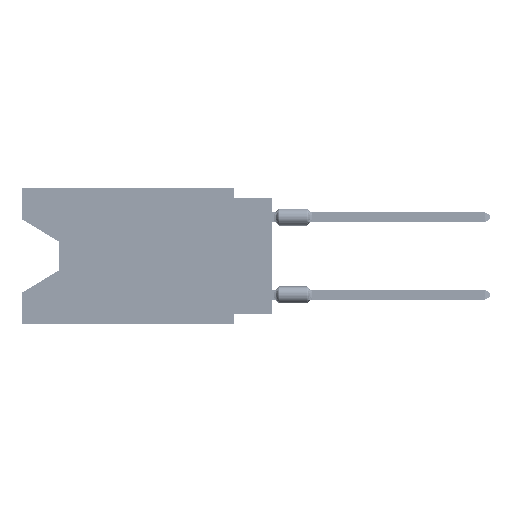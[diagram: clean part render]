
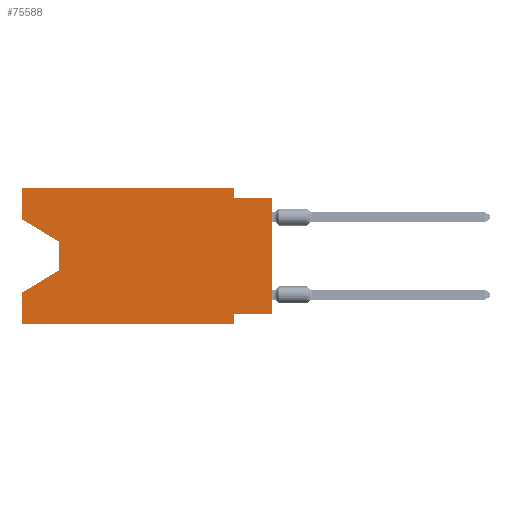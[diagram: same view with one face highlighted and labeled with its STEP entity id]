
A CAD part, left-side view. The second image highlights one B-rep face of the part: STEP entity #75588.
In plain terms, the highlighted planar face has unit normal (-1, 0, 0).
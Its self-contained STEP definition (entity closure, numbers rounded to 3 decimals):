
#758 = DIRECTION ( 'NONE',  ( 0., 0., -1. ) ) ;
#1873 = CARTESIAN_POINT ( 'NONE',  ( 0., 16.383, -8.89 ) ) ;
#2846 = ORIENTED_EDGE ( 'NONE', *, *, #29020, .F. ) ;
#3597 = LINE ( 'NONE', #11110, #65106 ) ;
#3714 = CARTESIAN_POINT ( 'NONE',  ( 0., 13.97, -5.385 ) ) ;
#6676 = VERTEX_POINT ( 'NONE', #95369 ) ;
#7500 = CARTESIAN_POINT ( 'NONE',  ( 0., 13.97, -3.505 ) ) ;
#9991 = CARTESIAN_POINT ( 'NONE',  ( 0., 16.383, 0. ) ) ;
#10137 = LINE ( 'NONE', #45891, #101192 ) ;
#11110 = CARTESIAN_POINT ( 'NONE',  ( 0., 16.383, -2.038 ) ) ;
#13546 = VERTEX_POINT ( 'NONE', #1873 ) ;
#13571 = CARTESIAN_POINT ( 'NONE',  ( 0., 16.383, -6.852 ) ) ;
#15167 = ORIENTED_EDGE ( 'NONE', *, *, #69775, .F. ) ;
#16075 = CARTESIAN_POINT ( 'NONE',  ( 0., 16.383, 0. ) ) ;
#16445 = EDGE_CURVE ( 'NONE', #98619, #56858, #60688, .T. ) ;
#16849 = DIRECTION ( 'NONE',  ( 0., 0., -1. ) ) ;
#18128 = ORIENTED_EDGE ( 'NONE', *, *, #16445, .T. ) ;
#18878 = DIRECTION ( 'NONE',  ( 0., 0., -1. ) ) ;
#21071 = DIRECTION ( 'NONE',  ( 0., 0., 1. ) ) ;
#21631 = VECTOR ( 'NONE', #18878, 1000. ) ;
#24177 = LINE ( 'NONE', #111835, #88287 ) ;
#24714 = DIRECTION ( 'NONE',  ( 0., -1., 0. ) ) ;
#25618 = VECTOR ( 'NONE', #24714, 1000. ) ;
#26440 = DIRECTION ( 'NONE',  ( 0., 0., 1. ) ) ;
#26732 = CARTESIAN_POINT ( 'NONE',  ( 0., 13.97, -5.385 ) ) ;
#27245 = CARTESIAN_POINT ( 'NONE',  ( 0., 16.383, 0. ) ) ;
#27459 = LINE ( 'NONE', #36098, #98020 ) ;
#29020 = EDGE_CURVE ( 'NONE', #13546, #40004, #30423, .T. ) ;
#30423 = LINE ( 'NONE', #41899, #40083 ) ;
#30498 = VERTEX_POINT ( 'NONE', #62076 ) ;
#30545 = EDGE_CURVE ( 'NONE', #84445, #42685, #10137, .T. ) ;
#30746 = VECTOR ( 'NONE', #26440, 1000. ) ;
#30876 = LINE ( 'NONE', #56811, #97747 ) ;
#34807 = ORIENTED_EDGE ( 'NONE', *, *, #102158, .T. ) ;
#36098 = CARTESIAN_POINT ( 'NONE',  ( 0., 0., -0.635 ) ) ;
#37066 = PLANE ( 'NONE',  #46306 ) ;
#37326 = EDGE_CURVE ( 'NONE', #68299, #98619, #3597, .T. ) ;
#37914 = VECTOR ( 'NONE', #95426, 1000. ) ;
#40004 = VERTEX_POINT ( 'NONE', #13571 ) ;
#40083 = VECTOR ( 'NONE', #101930, 1000. ) ;
#40901 = CARTESIAN_POINT ( 'NONE',  ( 0., 0., -0.635 ) ) ;
#41551 = EDGE_CURVE ( 'NONE', #68299, #113797, #50683, .T. ) ;
#41899 = CARTESIAN_POINT ( 'NONE',  ( 0., 16.383, 0. ) ) ;
#42685 = VERTEX_POINT ( 'NONE', #40901 ) ;
#44831 = VECTOR ( 'NONE', #16849, 1000. ) ;
#45407 = CARTESIAN_POINT ( 'NONE',  ( 0., 2.54, 0. ) ) ;
#45891 = CARTESIAN_POINT ( 'NONE',  ( 0., 0., 0. ) ) ;
#46096 = EDGE_CURVE ( 'NONE', #110345, #42685, #27459, .T. ) ;
#46296 = DIRECTION ( 'NONE',  ( 0., -0.855, -0.519 ) ) ;
#46306 = AXIS2_PLACEMENT_3D ( 'NONE', #9991, #90161, #758 ) ;
#50683 = LINE ( 'NONE', #16075, #30746 ) ;
#53201 = LINE ( 'NONE', #88431, #101116 ) ;
#56811 = CARTESIAN_POINT ( 'NONE',  ( 0., 2.54, -8.89 ) ) ;
#56858 = VERTEX_POINT ( 'NONE', #3714 ) ;
#56891 = ORIENTED_EDGE ( 'NONE', *, *, #66523, .T. ) ;
#60211 = LINE ( 'NONE', #26732, #37914 ) ;
#60212 = CARTESIAN_POINT ( 'NONE',  ( 0., 2.54, -0.635 ) ) ;
#60461 = VERTEX_POINT ( 'NONE', #82887 ) ;
#60688 = LINE ( 'NONE', #95908, #44831 ) ;
#62076 = CARTESIAN_POINT ( 'NONE',  ( 0., 2.54, -8.89 ) ) ;
#62352 = ORIENTED_EDGE ( 'NONE', *, *, #46096, .F. ) ;
#63884 = EDGE_CURVE ( 'NONE', #6676, #30498, #30876, .T. ) ;
#65106 = VECTOR ( 'NONE', #46296, 1000. ) ;
#66523 = EDGE_CURVE ( 'NONE', #56858, #40004, #60211, .T. ) ;
#68299 = VERTEX_POINT ( 'NONE', #82518 ) ;
#69775 = EDGE_CURVE ( 'NONE', #60461, #110345, #107678, .T. ) ;
#75588 = ADVANCED_FACE ( 'NONE', ( #81509 ), #37066, .F. ) ;
#77019 = EDGE_LOOP ( 'NONE', ( #101471, #18128, #56891, #2846, #34807, #110841, #83288, #77385, #62352, #15167, #92403, #94935 ) ) ;
#77385 = ORIENTED_EDGE ( 'NONE', *, *, #30545, .T. ) ;
#77781 = CARTESIAN_POINT ( 'NONE',  ( 0., 16.383, 0. ) ) ;
#80867 = EDGE_CURVE ( 'NONE', #84445, #6676, #53201, .T. ) ;
#81509 = FACE_OUTER_BOUND ( 'NONE', #77019, .T. ) ;
#82518 = CARTESIAN_POINT ( 'NONE',  ( 0., 16.383, -2.038 ) ) ;
#82887 = CARTESIAN_POINT ( 'NONE',  ( 0., 2.54, 0. ) ) ;
#83288 = ORIENTED_EDGE ( 'NONE', *, *, #80867, .F. ) ;
#84445 = VERTEX_POINT ( 'NONE', #107425 ) ;
#86438 = LINE ( 'NONE', #77781, #25618 ) ;
#87631 = DIRECTION ( 'NONE',  ( 0., -1., 0. ) ) ;
#88287 = VECTOR ( 'NONE', #87631, 1000. ) ;
#88431 = CARTESIAN_POINT ( 'NONE',  ( 0., 0., -8.255 ) ) ;
#90161 = DIRECTION ( 'NONE',  ( 1., 0., 0. ) ) ;
#90915 = EDGE_CURVE ( 'NONE', #113797, #60461, #86438, .T. ) ;
#91469 = DIRECTION ( 'NONE',  ( 0., 0., -1. ) ) ;
#92403 = ORIENTED_EDGE ( 'NONE', *, *, #90915, .F. ) ;
#94935 = ORIENTED_EDGE ( 'NONE', *, *, #41551, .F. ) ;
#95369 = CARTESIAN_POINT ( 'NONE',  ( 0., 2.54, -8.255 ) ) ;
#95426 = DIRECTION ( 'NONE',  ( 0., 0.855, -0.519 ) ) ;
#95908 = CARTESIAN_POINT ( 'NONE',  ( 0., 13.97, -3.505 ) ) ;
#97747 = VECTOR ( 'NONE', #91469, 1000. ) ;
#98020 = VECTOR ( 'NONE', #105358, 1000. ) ;
#98619 = VERTEX_POINT ( 'NONE', #7500 ) ;
#98761 = DIRECTION ( 'NONE',  ( 0., 1., 0. ) ) ;
#101116 = VECTOR ( 'NONE', #98761, 1000. ) ;
#101192 = VECTOR ( 'NONE', #21071, 1000. ) ;
#101471 = ORIENTED_EDGE ( 'NONE', *, *, #37326, .T. ) ;
#101930 = DIRECTION ( 'NONE',  ( 0., 0., 1. ) ) ;
#102158 = EDGE_CURVE ( 'NONE', #13546, #30498, #24177, .T. ) ;
#105358 = DIRECTION ( 'NONE',  ( 0., -1., 0. ) ) ;
#107425 = CARTESIAN_POINT ( 'NONE',  ( 0., 0., -8.255 ) ) ;
#107678 = LINE ( 'NONE', #45407, #21631 ) ;
#110345 = VERTEX_POINT ( 'NONE', #60212 ) ;
#110841 = ORIENTED_EDGE ( 'NONE', *, *, #63884, .F. ) ;
#111835 = CARTESIAN_POINT ( 'NONE',  ( 0., 16.383, -8.89 ) ) ;
#113797 = VERTEX_POINT ( 'NONE', #27245 ) ;
